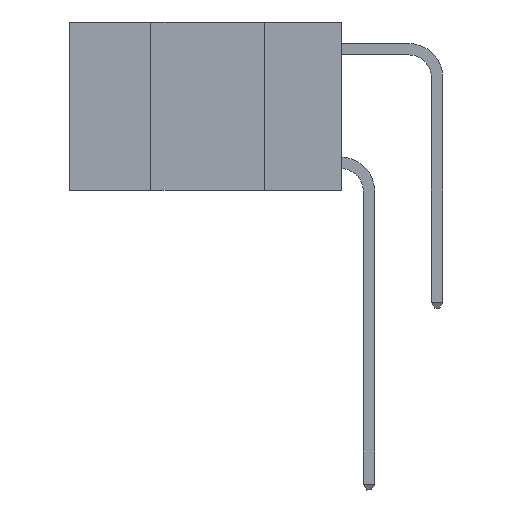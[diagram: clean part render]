
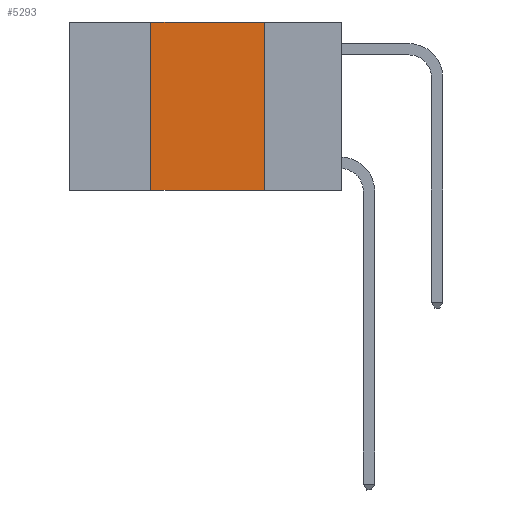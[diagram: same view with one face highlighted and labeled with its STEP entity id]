
A CAD part, left-side view. The second image highlights one B-rep face of the part: STEP entity #5293.
In plain terms, the highlighted planar face has unit normal (-1, 0, 0).
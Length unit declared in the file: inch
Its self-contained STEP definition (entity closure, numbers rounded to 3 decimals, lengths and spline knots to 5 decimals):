
#397 = VECTOR ( 'NONE', #3517, 39.37008 ) ;
#432 = VERTEX_POINT ( 'NONE', #6137 ) ;
#653 = VECTOR ( 'NONE', #12228, 39.37008 ) ;
#769 = VECTOR ( 'NONE', #7502, 39.37008 ) ;
#1066 = DIRECTION ( 'NONE',  ( 1., 0., 0. ) ) ;
#1322 = VERTEX_POINT ( 'NONE', #13167 ) ;
#1582 = EDGE_CURVE ( 'NONE', #1322, #11158, #3538, .T. ) ;
#1909 = FACE_OUTER_BOUND ( 'NONE', #12567, .T. ) ;
#2155 = CARTESIAN_POINT ( 'NONE',  ( 0., 0.6, 0. ) ) ;
#2234 = CARTESIAN_POINT ( 'NONE',  ( 0., 0.17, -0.37 ) ) ;
#2772 = ORIENTED_EDGE ( 'NONE', *, *, #1582, .F. ) ;
#2787 = ORIENTED_EDGE ( 'NONE', *, *, #10632, .F. ) ;
#3028 = ORIENTED_EDGE ( 'NONE', *, *, #3171, .F. ) ;
#3114 = ORIENTED_EDGE ( 'NONE', *, *, #4899, .T. ) ;
#3171 = EDGE_CURVE ( 'NONE', #6230, #432, #3649, .T. ) ;
#3517 = DIRECTION ( 'NONE',  ( 0., 0., 1. ) ) ;
#3538 = LINE ( 'NONE', #12177, #653 ) ;
#3649 = LINE ( 'NONE', #5588, #397 ) ;
#4156 = AXIS2_PLACEMENT_3D ( 'NONE', #2155, #1066, #8301 ) ;
#4899 = EDGE_CURVE ( 'NONE', #6230, #11158, #5750, .T. ) ;
#5293 = ADVANCED_FACE ( 'NONE', ( #1909 ), #8250, .F. ) ;
#5588 = CARTESIAN_POINT ( 'NONE',  ( 0., 0.42, 0. ) ) ;
#5750 = LINE ( 'NONE', #11700, #7418 ) ;
#6137 = CARTESIAN_POINT ( 'NONE',  ( 0., 0.42, 0. ) ) ;
#6230 = VERTEX_POINT ( 'NONE', #8797 ) ;
#7418 = VECTOR ( 'NONE', #11655, 39.37008 ) ;
#7502 = DIRECTION ( 'NONE',  ( 0., -1., 0. ) ) ;
#8250 = PLANE ( 'NONE',  #4156 ) ;
#8301 = DIRECTION ( 'NONE',  ( 0., 0., -1. ) ) ;
#8797 = CARTESIAN_POINT ( 'NONE',  ( 0., 0.42, -0.37 ) ) ;
#10616 = CARTESIAN_POINT ( 'NONE',  ( 0., 0.6, 0. ) ) ;
#10632 = EDGE_CURVE ( 'NONE', #432, #1322, #11766, .T. ) ;
#11158 = VERTEX_POINT ( 'NONE', #2234 ) ;
#11655 = DIRECTION ( 'NONE',  ( 0., -1., 0. ) ) ;
#11700 = CARTESIAN_POINT ( 'NONE',  ( 0., 0.6, -0.37 ) ) ;
#11766 = LINE ( 'NONE', #10616, #769 ) ;
#12177 = CARTESIAN_POINT ( 'NONE',  ( 0., 0.17, 0. ) ) ;
#12228 = DIRECTION ( 'NONE',  ( 0., 0., -1. ) ) ;
#12567 = EDGE_LOOP ( 'NONE', ( #2772, #2787, #3028, #3114 ) ) ;
#13167 = CARTESIAN_POINT ( 'NONE',  ( 0., 0.17, 0. ) ) ;
